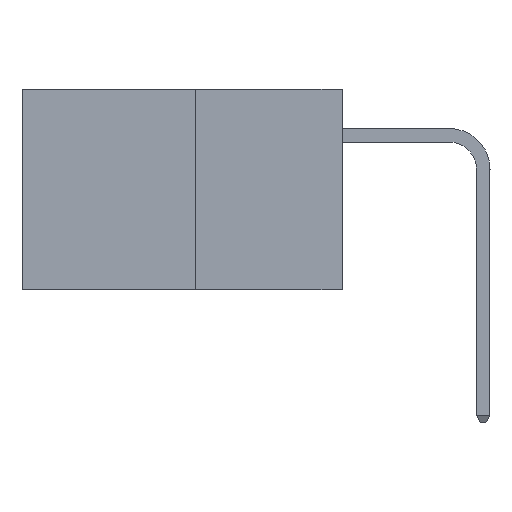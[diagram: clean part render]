
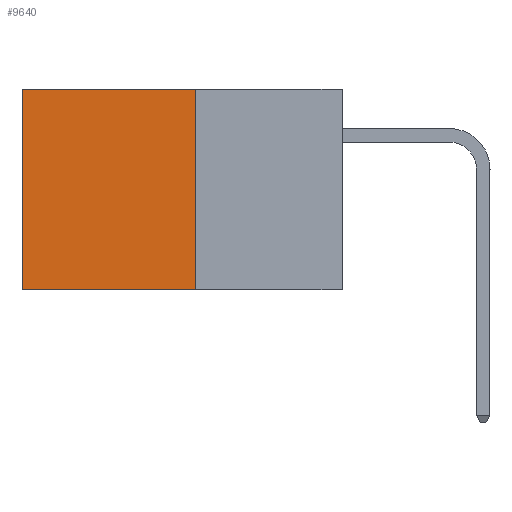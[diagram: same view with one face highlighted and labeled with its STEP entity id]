
A CAD part, left-side view. The second image highlights one B-rep face of the part: STEP entity #9640.
In plain terms, the highlighted planar face has unit normal (-1, 0, 0).
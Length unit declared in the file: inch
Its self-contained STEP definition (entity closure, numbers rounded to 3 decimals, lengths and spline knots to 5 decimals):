
#536 = DIRECTION ( 'NONE',  ( 0., 0., -1. ) ) ;
#1330 = EDGE_CURVE ( 'NONE', #7795, #8971, #3128, .T. ) ;
#1495 = EDGE_CURVE ( 'NONE', #7795, #12995, #13210, .T. ) ;
#1803 = AXIS2_PLACEMENT_3D ( 'NONE', #12093, #19440, #8485 ) ;
#1833 = VECTOR ( 'NONE', #536, 39.37008 ) ;
#3128 = LINE ( 'NONE', #9936, #12372 ) ;
#3919 = CARTESIAN_POINT ( 'NONE',  ( 0.277, 0.27, -0.37 ) ) ;
#4204 = CARTESIAN_POINT ( 'NONE',  ( 0.277, 0.59, 0. ) ) ;
#4620 = VERTEX_POINT ( 'NONE', #8670 ) ;
#5198 = ORIENTED_EDGE ( 'NONE', *, *, #1495, .T. ) ;
#5944 = LINE ( 'NONE', #3919, #15725 ) ;
#6784 = LINE ( 'NONE', #18832, #1833 ) ;
#7795 = VERTEX_POINT ( 'NONE', #8915 ) ;
#8335 = VECTOR ( 'NONE', #22433, 39.37008 ) ;
#8485 = DIRECTION ( 'NONE',  ( 0., 0., -1. ) ) ;
#8653 = EDGE_CURVE ( 'NONE', #12995, #4620, #6784, .T. ) ;
#8670 = CARTESIAN_POINT ( 'NONE',  ( 0.277, 0.59, -0.37 ) ) ;
#8915 = CARTESIAN_POINT ( 'NONE',  ( 0.277, 0.27, 0. ) ) ;
#8971 = VERTEX_POINT ( 'NONE', #14245 ) ;
#9640 = ADVANCED_FACE ( 'NONE', ( #10933 ), #17628, .F. ) ;
#9936 = CARTESIAN_POINT ( 'NONE',  ( 0.277, 0.27, -0.37 ) ) ;
#10099 = DIRECTION ( 'NONE',  ( 0., 0., -1. ) ) ;
#10152 = CARTESIAN_POINT ( 'NONE',  ( 0.277, 0.27, 0. ) ) ;
#10933 = FACE_OUTER_BOUND ( 'NONE', #11752, .T. ) ;
#11752 = EDGE_LOOP ( 'NONE', ( #20836, #18278, #12348, #5198 ) ) ;
#12093 = CARTESIAN_POINT ( 'NONE',  ( 0.277, 0.27, -0.37 ) ) ;
#12348 = ORIENTED_EDGE ( 'NONE', *, *, #1330, .F. ) ;
#12372 = VECTOR ( 'NONE', #10099, 39.37008 ) ;
#12995 = VERTEX_POINT ( 'NONE', #4204 ) ;
#13210 = LINE ( 'NONE', #10152, #8335 ) ;
#14245 = CARTESIAN_POINT ( 'NONE',  ( 0.277, 0.27, -0.37 ) ) ;
#14980 = DIRECTION ( 'NONE',  ( 0., 1., 0. ) ) ;
#15725 = VECTOR ( 'NONE', #14980, 39.37008 ) ;
#17628 = PLANE ( 'NONE',  #1803 ) ;
#18278 = ORIENTED_EDGE ( 'NONE', *, *, #19407, .F. ) ;
#18832 = CARTESIAN_POINT ( 'NONE',  ( 0.277, 0.59, -0.37 ) ) ;
#19407 = EDGE_CURVE ( 'NONE', #8971, #4620, #5944, .T. ) ;
#19440 = DIRECTION ( 'NONE',  ( 1., 0., 0. ) ) ;
#20836 = ORIENTED_EDGE ( 'NONE', *, *, #8653, .T. ) ;
#22433 = DIRECTION ( 'NONE',  ( 0., 1., 0. ) ) ;
